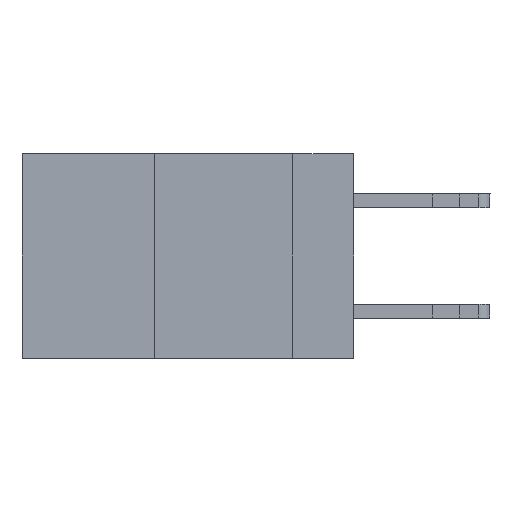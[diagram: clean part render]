
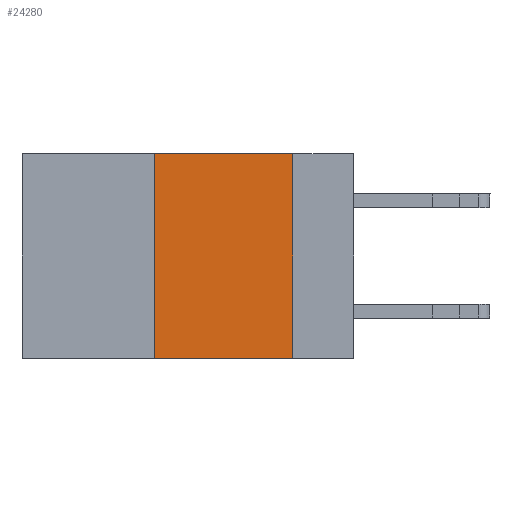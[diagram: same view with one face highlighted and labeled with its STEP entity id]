
A CAD part, left-side view. The second image highlights one B-rep face of the part: STEP entity #24280.
In plain terms, the highlighted planar face has unit normal (-1, 0, 0).
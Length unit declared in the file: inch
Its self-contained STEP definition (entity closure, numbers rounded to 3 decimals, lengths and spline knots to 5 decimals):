
#726 = ORIENTED_EDGE ( 'NONE', *, *, #20555, .F. ) ;
#847 = VERTEX_POINT ( 'NONE', #20659 ) ;
#887 = CARTESIAN_POINT ( 'NONE',  ( 0., 0.11, -0.37 ) ) ;
#1036 = DIRECTION ( 'NONE',  ( 0., -1., 0. ) ) ;
#2063 = LINE ( 'NONE', #7679, #3340 ) ;
#2386 = ORIENTED_EDGE ( 'NONE', *, *, #22172, .F. ) ;
#3340 = VECTOR ( 'NONE', #11663, 39.37008 ) ;
#3460 = LINE ( 'NONE', #22742, #13452 ) ;
#3928 = CARTESIAN_POINT ( 'NONE',  ( 0., 0.6, 0. ) ) ;
#4375 = VERTEX_POINT ( 'NONE', #18787 ) ;
#4886 = EDGE_CURVE ( 'NONE', #847, #11288, #3460, .T. ) ;
#5965 = DIRECTION ( 'NONE',  ( 0., 0., -1. ) ) ;
#7679 = CARTESIAN_POINT ( 'NONE',  ( 0., 0.36, 0. ) ) ;
#8200 = LINE ( 'NONE', #8512, #18176 ) ;
#8512 = CARTESIAN_POINT ( 'NONE',  ( 0., 0.11, 0. ) ) ;
#8848 = DIRECTION ( 'NONE',  ( 0., -1., 0. ) ) ;
#9005 = AXIS2_PLACEMENT_3D ( 'NONE', #3928, #17867, #5965 ) ;
#9748 = PLANE ( 'NONE',  #9005 ) ;
#11034 = CARTESIAN_POINT ( 'NONE',  ( 0., 0.6, 0. ) ) ;
#11288 = VERTEX_POINT ( 'NONE', #887 ) ;
#11663 = DIRECTION ( 'NONE',  ( 0., 0., 1. ) ) ;
#11813 = ORIENTED_EDGE ( 'NONE', *, *, #12351, .F. ) ;
#12351 = EDGE_CURVE ( 'NONE', #20082, #11288, #8200, .T. ) ;
#13452 = VECTOR ( 'NONE', #8848, 39.37008 ) ;
#14068 = LINE ( 'NONE', #11034, #18730 ) ;
#14476 = FACE_OUTER_BOUND ( 'NONE', #14545, .T. ) ;
#14545 = EDGE_LOOP ( 'NONE', ( #11813, #726, #2386, #17462 ) ) ;
#15651 = CARTESIAN_POINT ( 'NONE',  ( 0., 0.11, 0. ) ) ;
#17462 = ORIENTED_EDGE ( 'NONE', *, *, #4886, .T. ) ;
#17867 = DIRECTION ( 'NONE',  ( 1., 0., 0. ) ) ;
#18176 = VECTOR ( 'NONE', #20276, 39.37008 ) ;
#18730 = VECTOR ( 'NONE', #1036, 39.37008 ) ;
#18787 = CARTESIAN_POINT ( 'NONE',  ( 0., 0.36, 0. ) ) ;
#20082 = VERTEX_POINT ( 'NONE', #15651 ) ;
#20276 = DIRECTION ( 'NONE',  ( 0., 0., -1. ) ) ;
#20555 = EDGE_CURVE ( 'NONE', #4375, #20082, #14068, .T. ) ;
#20659 = CARTESIAN_POINT ( 'NONE',  ( 0., 0.36, -0.37 ) ) ;
#22172 = EDGE_CURVE ( 'NONE', #847, #4375, #2063, .T. ) ;
#22742 = CARTESIAN_POINT ( 'NONE',  ( 0., 0.6, -0.37 ) ) ;
#24280 = ADVANCED_FACE ( 'NONE', ( #14476 ), #9748, .F. ) ;
